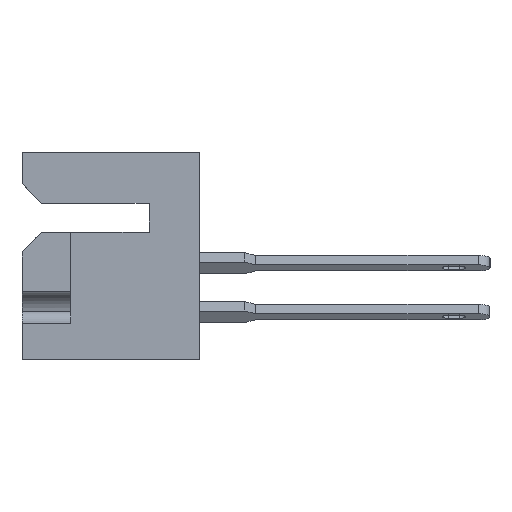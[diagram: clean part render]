
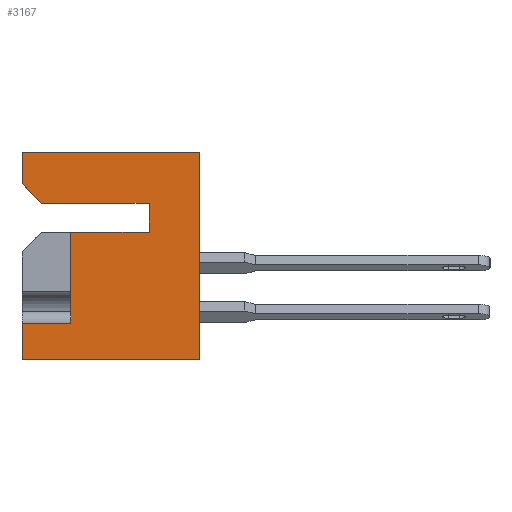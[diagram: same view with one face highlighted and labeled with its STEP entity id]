
A CAD part, left-side view. The second image highlights one B-rep face of the part: STEP entity #3167.
In plain terms, the highlighted planar face has unit normal (-1, 0, 0).
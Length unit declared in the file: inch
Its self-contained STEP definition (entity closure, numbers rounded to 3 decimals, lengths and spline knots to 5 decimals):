
#38 = LINE ( 'NONE', #4636, #14408 ) ;
#302 = ORIENTED_EDGE ( 'NONE', *, *, #5015, .T. ) ;
#341 = CARTESIAN_POINT ( 'NONE',  ( 0., 0.453, -0.081 ) ) ;
#779 = PLANE ( 'NONE',  #14448 ) ;
#2074 = CARTESIAN_POINT ( 'NONE',  ( 0., 0.403, -0.131 ) ) ;
#2746 = VECTOR ( 'NONE', #5503, 39.37008 ) ;
#2824 = VERTEX_POINT ( 'NONE', #8678 ) ;
#3002 = VERTEX_POINT ( 'NONE', #341 ) ;
#3019 = DIRECTION ( 'NONE',  ( 0., 0., 1. ) ) ;
#3167 = ADVANCED_FACE ( 'NONE', ( #3973 ), #779, .F. ) ;
#3440 = VERTEX_POINT ( 'NONE', #5675 ) ;
#3973 = FACE_OUTER_BOUND ( 'NONE', #4170, .T. ) ;
#3990 = LINE ( 'NONE', #2074, #13570 ) ;
#4099 = EDGE_CURVE ( 'NONE', #3002, #9319, #14326, .T. ) ;
#4170 = EDGE_LOOP ( 'NONE', ( #14116, #14955, #14447, #11489, #13500, #13004, #6196, #15490, #11626, #302, #11825 ) ) ;
#4296 = LINE ( 'NONE', #15589, #10097 ) ;
#4322 = VERTEX_POINT ( 'NONE', #16320 ) ;
#4513 = LINE ( 'NONE', #4897, #8101 ) ;
#4636 = CARTESIAN_POINT ( 'NONE',  ( 0., 0.328, -0.205 ) ) ;
#4697 = CARTESIAN_POINT ( 'NONE',  ( 0., 0., 0. ) ) ;
#4897 = CARTESIAN_POINT ( 'NONE',  ( 0., 0.128, -0.205 ) ) ;
#4956 = CARTESIAN_POINT ( 'NONE',  ( 0., 0.128, -0.131 ) ) ;
#5015 = EDGE_CURVE ( 'NONE', #14808, #4322, #4513, .T. ) ;
#5503 = DIRECTION ( 'NONE',  ( 0., 0., 1. ) ) ;
#5675 = CARTESIAN_POINT ( 'NONE',  ( 0., 0., -0.531 ) ) ;
#5692 = DIRECTION ( 'NONE',  ( 1., 0., 0. ) ) ;
#5806 = DIRECTION ( 'NONE',  ( 0., 0., 1. ) ) ;
#5879 = CARTESIAN_POINT ( 'NONE',  ( 0., 0.403, -0.131 ) ) ;
#5957 = DIRECTION ( 'NONE',  ( 0., 1., 0. ) ) ;
#6024 = EDGE_CURVE ( 'NONE', #2824, #3440, #12452, .T. ) ;
#6196 = ORIENTED_EDGE ( 'NONE', *, *, #12717, .T. ) ;
#6739 = CARTESIAN_POINT ( 'NONE',  ( 0., 0.453, -0.531 ) ) ;
#6931 = CARTESIAN_POINT ( 'NONE',  ( 0., 0.453, 0. ) ) ;
#7022 = CARTESIAN_POINT ( 'NONE',  ( 0., 0.453, 0. ) ) ;
#7126 = DIRECTION ( 'NONE',  ( 0., -0.707, -0.707 ) ) ;
#7198 = CARTESIAN_POINT ( 'NONE',  ( 0., 0., 0. ) ) ;
#7250 = DIRECTION ( 'NONE',  ( 0., 0., 1. ) ) ;
#7452 = CARTESIAN_POINT ( 'NONE',  ( 0., 0.453, 0. ) ) ;
#7650 = CARTESIAN_POINT ( 'NONE',  ( 0., 0.328, -0.437 ) ) ;
#8101 = VECTOR ( 'NONE', #5957, 39.37008 ) ;
#8372 = DIRECTION ( 'NONE',  ( 0., 0., -1. ) ) ;
#8675 = VERTEX_POINT ( 'NONE', #8908 ) ;
#8678 = CARTESIAN_POINT ( 'NONE',  ( 0., 0.453, -0.531 ) ) ;
#8725 = LINE ( 'NONE', #7198, #13727 ) ;
#8791 = DIRECTION ( 'NONE',  ( 0., -1., 0. ) ) ;
#8908 = CARTESIAN_POINT ( 'NONE',  ( 0., 0.453, -0.437 ) ) ;
#8983 = EDGE_CURVE ( 'NONE', #3440, #9790, #8725, .T. ) ;
#9265 = VERTEX_POINT ( 'NONE', #13651 ) ;
#9319 = VERTEX_POINT ( 'NONE', #10297 ) ;
#9386 = VECTOR ( 'NONE', #8791, 39.37008 ) ;
#9416 = VECTOR ( 'NONE', #11540, 39.37008 ) ;
#9535 = EDGE_CURVE ( 'NONE', #2824, #8675, #4296, .T. ) ;
#9584 = VERTEX_POINT ( 'NONE', #13245 ) ;
#9790 = VERTEX_POINT ( 'NONE', #4697 ) ;
#10097 = VECTOR ( 'NONE', #3019, 39.37008 ) ;
#10209 = CARTESIAN_POINT ( 'NONE',  ( 0., 0.128, -0.205 ) ) ;
#10297 = CARTESIAN_POINT ( 'NONE',  ( 0., 0.453, 0. ) ) ;
#10998 = VERTEX_POINT ( 'NONE', #5879 ) ;
#11489 = ORIENTED_EDGE ( 'NONE', *, *, #8983, .T. ) ;
#11540 = DIRECTION ( 'NONE',  ( 0., 1., 0. ) ) ;
#11599 = LINE ( 'NONE', #14063, #12601 ) ;
#11626 = ORIENTED_EDGE ( 'NONE', *, *, #15857, .F. ) ;
#11763 = EDGE_CURVE ( 'NONE', #9265, #10998, #12801, .T. ) ;
#11825 = ORIENTED_EDGE ( 'NONE', *, *, #15686, .F. ) ;
#12397 = EDGE_CURVE ( 'NONE', #9584, #8675, #13588, .T. ) ;
#12452 = LINE ( 'NONE', #6739, #14454 ) ;
#12601 = VECTOR ( 'NONE', #12720, 39.37008 ) ;
#12717 = EDGE_CURVE ( 'NONE', #3002, #10998, #3990, .T. ) ;
#12720 = DIRECTION ( 'NONE',  ( 0., 0., 1. ) ) ;
#12801 = LINE ( 'NONE', #4956, #9416 ) ;
#13004 = ORIENTED_EDGE ( 'NONE', *, *, #4099, .F. ) ;
#13189 = VECTOR ( 'NONE', #16367, 39.37008 ) ;
#13245 = CARTESIAN_POINT ( 'NONE',  ( 0., 0.328, -0.437 ) ) ;
#13500 = ORIENTED_EDGE ( 'NONE', *, *, #13601, .F. ) ;
#13570 = VECTOR ( 'NONE', #7126, 39.37008 ) ;
#13588 = LINE ( 'NONE', #7650, #13189 ) ;
#13601 = EDGE_CURVE ( 'NONE', #9319, #9790, #15154, .T. ) ;
#13651 = CARTESIAN_POINT ( 'NONE',  ( 0., 0.128, -0.131 ) ) ;
#13727 = VECTOR ( 'NONE', #5806, 39.37008 ) ;
#14063 = CARTESIAN_POINT ( 'NONE',  ( 0., 0.128, -0.131 ) ) ;
#14116 = ORIENTED_EDGE ( 'NONE', *, *, #12397, .T. ) ;
#14326 = LINE ( 'NONE', #6931, #2746 ) ;
#14408 = VECTOR ( 'NONE', #7250, 39.37008 ) ;
#14447 = ORIENTED_EDGE ( 'NONE', *, *, #6024, .T. ) ;
#14448 = AXIS2_PLACEMENT_3D ( 'NONE', #7022, #5692, #8372 ) ;
#14454 = VECTOR ( 'NONE', #15705, 39.37008 ) ;
#14808 = VERTEX_POINT ( 'NONE', #10209 ) ;
#14955 = ORIENTED_EDGE ( 'NONE', *, *, #9535, .F. ) ;
#15154 = LINE ( 'NONE', #7452, #9386 ) ;
#15490 = ORIENTED_EDGE ( 'NONE', *, *, #11763, .F. ) ;
#15589 = CARTESIAN_POINT ( 'NONE',  ( 0., 0.453, 0. ) ) ;
#15686 = EDGE_CURVE ( 'NONE', #9584, #4322, #38, .T. ) ;
#15705 = DIRECTION ( 'NONE',  ( 0., -1., 0. ) ) ;
#15857 = EDGE_CURVE ( 'NONE', #14808, #9265, #11599, .T. ) ;
#16320 = CARTESIAN_POINT ( 'NONE',  ( 0., 0.328, -0.205 ) ) ;
#16367 = DIRECTION ( 'NONE',  ( 0., 1., 0. ) ) ;
